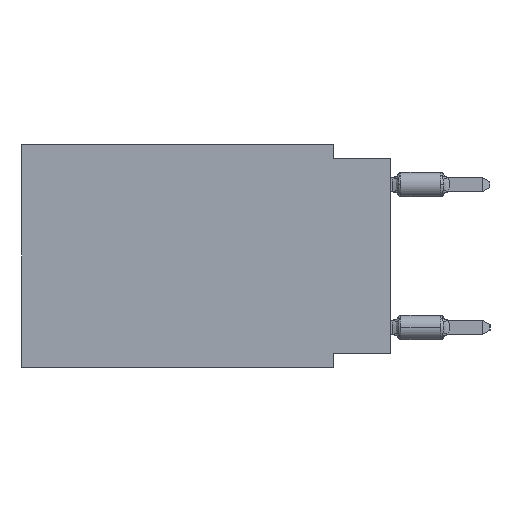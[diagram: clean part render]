
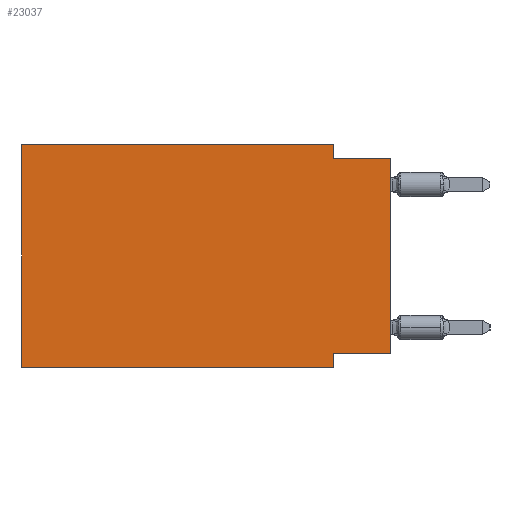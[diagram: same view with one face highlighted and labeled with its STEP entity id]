
A CAD part, left-side view. The second image highlights one B-rep face of the part: STEP entity #23037.
In plain terms, the highlighted planar face has unit normal (-1, 0, 0).
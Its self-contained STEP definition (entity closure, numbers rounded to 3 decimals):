
#163 = CARTESIAN_POINT ( 'NONE',  ( 0., 2.54, 0. ) ) ;
#482 = DIRECTION ( 'NONE',  ( 0., 0., 1. ) ) ;
#658 = EDGE_CURVE ( 'NONE', #1750, #38923, #33534, .T. ) ;
#1236 = VECTOR ( 'NONE', #38744, 1000. ) ;
#1323 = LINE ( 'NONE', #1809, #35075 ) ;
#1750 = VERTEX_POINT ( 'NONE', #35543 ) ;
#1809 = CARTESIAN_POINT ( 'NONE',  ( 0., 2.54, -9.906 ) ) ;
#3308 = LINE ( 'NONE', #25702, #28383 ) ;
#3770 = DIRECTION ( 'NONE',  ( 0., 1., 0. ) ) ;
#6171 = VERTEX_POINT ( 'NONE', #19769 ) ;
#6785 = DIRECTION ( 'NONE',  ( 0., 0., -1. ) ) ;
#7178 = CARTESIAN_POINT ( 'NONE',  ( 0., 16.383, 0. ) ) ;
#7906 = VERTEX_POINT ( 'NONE', #10184 ) ;
#8072 = VECTOR ( 'NONE', #482, 1000. ) ;
#9489 = ORIENTED_EDGE ( 'NONE', *, *, #658, .F. ) ;
#9632 = CARTESIAN_POINT ( 'NONE',  ( 0., 16.383, -9.906 ) ) ;
#9941 = PLANE ( 'NONE',  #31199 ) ;
#10160 = VECTOR ( 'NONE', #25879, 1000. ) ;
#10184 = CARTESIAN_POINT ( 'NONE',  ( 0., 16.383, 0. ) ) ;
#10574 = CARTESIAN_POINT ( 'NONE',  ( 0., 2.54, -9.271 ) ) ;
#10819 = LINE ( 'NONE', #7178, #32133 ) ;
#11024 = CARTESIAN_POINT ( 'NONE',  ( 0., 0., -0.635 ) ) ;
#11169 = ORIENTED_EDGE ( 'NONE', *, *, #31227, .F. ) ;
#11763 = ORIENTED_EDGE ( 'NONE', *, *, #20407, .T. ) ;
#12621 = DIRECTION ( 'NONE',  ( 0., 0., 1. ) ) ;
#12808 = ORIENTED_EDGE ( 'NONE', *, *, #22778, .F. ) ;
#13022 = DIRECTION ( 'NONE',  ( 0., 0., -1. ) ) ;
#14243 = ORIENTED_EDGE ( 'NONE', *, *, #17358, .F. ) ;
#14462 = CARTESIAN_POINT ( 'NONE',  ( 0., 0., -9.271 ) ) ;
#14660 = LINE ( 'NONE', #11024, #10160 ) ;
#15491 = EDGE_CURVE ( 'NONE', #30393, #6171, #1323, .T. ) ;
#15541 = CARTESIAN_POINT ( 'NONE',  ( 0., 0., -0.635 ) ) ;
#15598 = VECTOR ( 'NONE', #6785, 1000. ) ;
#16257 = LINE ( 'NONE', #31117, #45087 ) ;
#17080 = VERTEX_POINT ( 'NONE', #9632 ) ;
#17358 = EDGE_CURVE ( 'NONE', #7906, #1750, #10819, .T. ) ;
#17491 = DIRECTION ( 'NONE',  ( 1., 0., 0. ) ) ;
#19769 = CARTESIAN_POINT ( 'NONE',  ( 0., 2.54, -9.906 ) ) ;
#20287 = ORIENTED_EDGE ( 'NONE', *, *, #32018, .T. ) ;
#20407 = EDGE_CURVE ( 'NONE', #42472, #25707, #16257, .T. ) ;
#22019 = DIRECTION ( 'NONE',  ( 0., -1., 0. ) ) ;
#22778 = EDGE_CURVE ( 'NONE', #38923, #25707, #14660, .T. ) ;
#23037 = ADVANCED_FACE ( 'NONE', ( #36258 ), #9941, .F. ) ;
#23864 = LINE ( 'NONE', #28247, #1236 ) ;
#25702 = CARTESIAN_POINT ( 'NONE',  ( 0., 0., -9.271 ) ) ;
#25707 = VERTEX_POINT ( 'NONE', #15541 ) ;
#25879 = DIRECTION ( 'NONE',  ( 0., -1., 0. ) ) ;
#27022 = LINE ( 'NONE', #45325, #8072 ) ;
#28247 = CARTESIAN_POINT ( 'NONE',  ( 0., 16.383, -9.906 ) ) ;
#28383 = VECTOR ( 'NONE', #3770, 1000. ) ;
#29211 = EDGE_CURVE ( 'NONE', #17080, #7906, #27022, .T. ) ;
#30393 = VERTEX_POINT ( 'NONE', #10574 ) ;
#31117 = CARTESIAN_POINT ( 'NONE',  ( 0., 0., 0. ) ) ;
#31199 = AXIS2_PLACEMENT_3D ( 'NONE', #43322, #17491, #43545 ) ;
#31227 = EDGE_CURVE ( 'NONE', #42472, #30393, #3308, .T. ) ;
#32018 = EDGE_CURVE ( 'NONE', #17080, #6171, #23864, .T. ) ;
#32133 = VECTOR ( 'NONE', #22019, 1000. ) ;
#33534 = LINE ( 'NONE', #163, #15598 ) ;
#34287 = CARTESIAN_POINT ( 'NONE',  ( 0., 2.54, -0.635 ) ) ;
#35075 = VECTOR ( 'NONE', #13022, 1000. ) ;
#35197 = EDGE_LOOP ( 'NONE', ( #11763, #12808, #9489, #14243, #41791, #20287, #47796, #11169 ) ) ;
#35543 = CARTESIAN_POINT ( 'NONE',  ( 0., 2.54, 0. ) ) ;
#36258 = FACE_OUTER_BOUND ( 'NONE', #35197, .T. ) ;
#38744 = DIRECTION ( 'NONE',  ( 0., -1., 0. ) ) ;
#38923 = VERTEX_POINT ( 'NONE', #34287 ) ;
#41791 = ORIENTED_EDGE ( 'NONE', *, *, #29211, .F. ) ;
#42472 = VERTEX_POINT ( 'NONE', #14462 ) ;
#43322 = CARTESIAN_POINT ( 'NONE',  ( 0., 16.383, 0. ) ) ;
#43545 = DIRECTION ( 'NONE',  ( 0., 0., -1. ) ) ;
#45087 = VECTOR ( 'NONE', #12621, 1000. ) ;
#45325 = CARTESIAN_POINT ( 'NONE',  ( 0., 16.383, 0. ) ) ;
#47796 = ORIENTED_EDGE ( 'NONE', *, *, #15491, .F. ) ;
